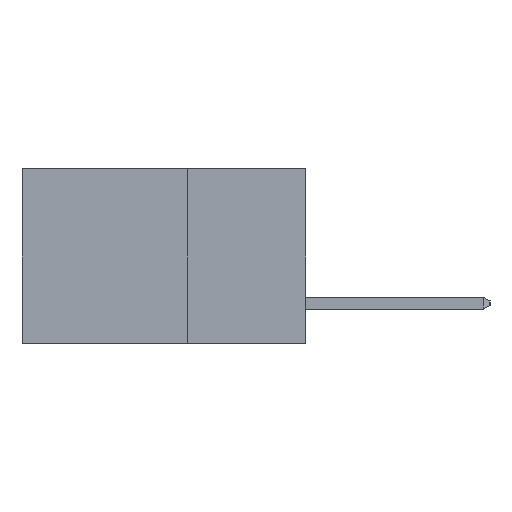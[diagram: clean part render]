
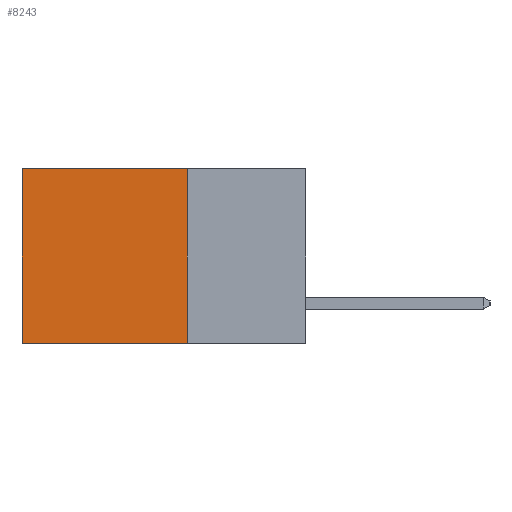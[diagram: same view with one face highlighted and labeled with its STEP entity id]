
A CAD part, left-side view. The second image highlights one B-rep face of the part: STEP entity #8243.
In plain terms, the highlighted planar face has unit normal (-1, 0, 0).
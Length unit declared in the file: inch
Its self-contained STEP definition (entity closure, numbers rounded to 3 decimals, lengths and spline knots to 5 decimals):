
#759 = PLANE ( 'NONE',  #7464 ) ;
#1366 = CARTESIAN_POINT ( 'NONE',  ( 0.2615, 0.6, 0. ) ) ;
#1472 = CARTESIAN_POINT ( 'NONE',  ( 0.2615, 0.25, 0. ) ) ;
#1545 = DIRECTION ( 'NONE',  ( 1., 0., 0. ) ) ;
#1558 = DIRECTION ( 'NONE',  ( 0., 0., -1. ) ) ;
#1672 = LINE ( 'NONE', #4527, #9204 ) ;
#2141 = CARTESIAN_POINT ( 'NONE',  ( 0.2615, 0.25, 0. ) ) ;
#2158 = CARTESIAN_POINT ( 'NONE',  ( 0.2615, 0.6, -0.37 ) ) ;
#2304 = FACE_OUTER_BOUND ( 'NONE', #3060, .T. ) ;
#2684 = EDGE_CURVE ( 'NONE', #5866, #7611, #9015, .T. ) ;
#2984 = LINE ( 'NONE', #6628, #4260 ) ;
#3060 = EDGE_LOOP ( 'NONE', ( #4898, #4555, #4350, #8555 ) ) ;
#3749 = VERTEX_POINT ( 'NONE', #6561 ) ;
#3782 = VECTOR ( 'NONE', #6637, 39.37008 ) ;
#4260 = VECTOR ( 'NONE', #4396, 39.37008 ) ;
#4350 = ORIENTED_EDGE ( 'NONE', *, *, #9352, .F. ) ;
#4356 = DIRECTION ( 'NONE',  ( 0., 0., -1. ) ) ;
#4396 = DIRECTION ( 'NONE',  ( 0., 1., 0. ) ) ;
#4408 = CARTESIAN_POINT ( 'NONE',  ( 0.2615, 0.6, -0.37 ) ) ;
#4527 = CARTESIAN_POINT ( 'NONE',  ( 0.2615, 0.25, -0.37 ) ) ;
#4555 = ORIENTED_EDGE ( 'NONE', *, *, #7159, .F. ) ;
#4898 = ORIENTED_EDGE ( 'NONE', *, *, #2684, .T. ) ;
#5866 = VERTEX_POINT ( 'NONE', #1366 ) ;
#5945 = VERTEX_POINT ( 'NONE', #1472 ) ;
#6025 = LINE ( 'NONE', #2141, #3782 ) ;
#6039 = CARTESIAN_POINT ( 'NONE',  ( 0.2615, 0.25, -0.37 ) ) ;
#6561 = CARTESIAN_POINT ( 'NONE',  ( 0.2615, 0.25, -0.37 ) ) ;
#6628 = CARTESIAN_POINT ( 'NONE',  ( 0.2615, 0.25, -0.37 ) ) ;
#6637 = DIRECTION ( 'NONE',  ( 0., 1., 0. ) ) ;
#6772 = DIRECTION ( 'NONE',  ( 0., 0., -1. ) ) ;
#7159 = EDGE_CURVE ( 'NONE', #3749, #7611, #2984, .T. ) ;
#7464 = AXIS2_PLACEMENT_3D ( 'NONE', #6039, #1545, #6772 ) ;
#7611 = VERTEX_POINT ( 'NONE', #2158 ) ;
#8243 = ADVANCED_FACE ( 'NONE', ( #2304 ), #759, .F. ) ;
#8555 = ORIENTED_EDGE ( 'NONE', *, *, #8703, .T. ) ;
#8703 = EDGE_CURVE ( 'NONE', #5945, #5866, #6025, .T. ) ;
#8804 = VECTOR ( 'NONE', #4356, 39.37008 ) ;
#9015 = LINE ( 'NONE', #4408, #8804 ) ;
#9204 = VECTOR ( 'NONE', #1558, 39.37008 ) ;
#9352 = EDGE_CURVE ( 'NONE', #5945, #3749, #1672, .T. ) ;
